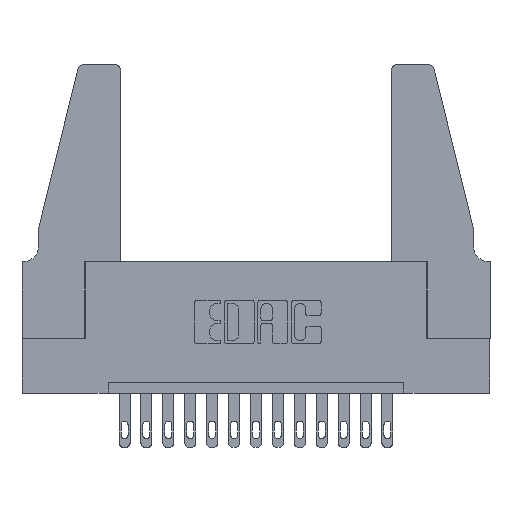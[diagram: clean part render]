
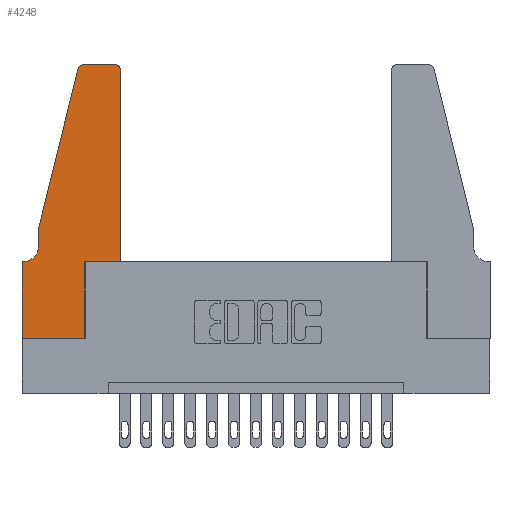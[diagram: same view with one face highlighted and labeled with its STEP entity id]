
A CAD part, top view. The second image highlights one B-rep face of the part: STEP entity #4248.
In plain terms, the highlighted planar face has unit normal (0, 0, 1).
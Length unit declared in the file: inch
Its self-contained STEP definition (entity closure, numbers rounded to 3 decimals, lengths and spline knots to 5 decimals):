
#276 = EDGE_CURVE ( 'NONE', #4902, #3095, #9481, .T. ) ;
#362 = CARTESIAN_POINT ( 'NONE',  ( 0.2605, 1.25, 0.37 ) ) ;
#485 = DIRECTION ( 'NONE',  ( 1., 0., 0. ) ) ;
#651 = CARTESIAN_POINT ( 'NONE',  ( 0.4505, 0.35, 0.37 ) ) ;
#668 = LINE ( 'NONE', #13694, #14025 ) ;
#690 = VECTOR ( 'NONE', #12337, 39.37008 ) ;
#999 = CARTESIAN_POINT ( 'NONE',  ( 0., 0., 0.37 ) ) ;
#1260 = CARTESIAN_POINT ( 'NONE',  ( 0.284, 1.25, 0.37 ) ) ;
#1362 = DIRECTION ( 'NONE',  ( 0., 0., 1. ) ) ;
#1658 = VERTEX_POINT ( 'NONE', #10302 ) ;
#1720 = ORIENTED_EDGE ( 'NONE', *, *, #7773, .T. ) ;
#1748 = VERTEX_POINT ( 'NONE', #2417 ) ;
#2011 = VECTOR ( 'NONE', #13747, 39.37008 ) ;
#2058 = VERTEX_POINT ( 'NONE', #1260 ) ;
#2111 = ORIENTED_EDGE ( 'NONE', *, *, #12207, .T. ) ;
#2129 = DIRECTION ( 'NONE',  ( 0., -1., 0. ) ) ;
#2417 = CARTESIAN_POINT ( 'NONE',  ( 0.0755, 0.5, 0.37 ) ) ;
#2458 = CARTESIAN_POINT ( 'NONE',  ( 0.2865, 0.35, 0.37 ) ) ;
#2506 = VERTEX_POINT ( 'NONE', #999 ) ;
#2629 = ORIENTED_EDGE ( 'NONE', *, *, #15460, .T. ) ;
#2761 = VERTEX_POINT ( 'NONE', #12954 ) ;
#2766 = AXIS2_PLACEMENT_3D ( 'NONE', #8630, #1362, #9855 ) ;
#3017 = AXIS2_PLACEMENT_3D ( 'NONE', #14844, #3873, #13804 ) ;
#3095 = VERTEX_POINT ( 'NONE', #2458 ) ;
#3340 = DIRECTION ( 'NONE',  ( 0., 1., 0. ) ) ;
#3521 = CARTESIAN_POINT ( 'NONE',  ( 0.0755, 0.5, 0.37 ) ) ;
#3535 = ORIENTED_EDGE ( 'NONE', *, *, #276, .T. ) ;
#3569 = ORIENTED_EDGE ( 'NONE', *, *, #9164, .T. ) ;
#3797 = VECTOR ( 'NONE', #12333, 39.37008 ) ;
#3873 = DIRECTION ( 'NONE',  ( 0., 0., -1. ) ) ;
#3899 = EDGE_CURVE ( 'NONE', #2506, #4902, #15775, .T. ) ;
#3939 = VECTOR ( 'NONE', #2129, 39.37008 ) ;
#4248 = ADVANCED_FACE ( 'NONE', ( #6786 ), #12271, .T. ) ;
#4289 = LINE ( 'NONE', #4987, #690 ) ;
#4370 = ORIENTED_EDGE ( 'NONE', *, *, #4925, .T. ) ;
#4902 = VERTEX_POINT ( 'NONE', #9717 ) ;
#4925 = EDGE_CURVE ( 'NONE', #12838, #2506, #4289, .T. ) ;
#4987 = CARTESIAN_POINT ( 'NONE',  ( 0., 0., 0.37 ) ) ;
#5018 = ORIENTED_EDGE ( 'NONE', *, *, #11725, .T. ) ;
#5132 = ORIENTED_EDGE ( 'NONE', *, *, #5438, .T. ) ;
#5137 = CIRCLE ( 'NONE', #13045, 0.03 ) ;
#5313 = CARTESIAN_POINT ( 'NONE',  ( 0.0755, 0.42, 0.37 ) ) ;
#5438 = EDGE_CURVE ( 'NONE', #15769, #1748, #11888, .T. ) ;
#5461 = LINE ( 'NONE', #9497, #3939 ) ;
#5871 = CARTESIAN_POINT ( 'NONE',  ( 0.2865, 0.35, 0.37 ) ) ;
#6216 = CARTESIAN_POINT ( 'NONE',  ( 0.0755, 0.35, 0.37 ) ) ;
#6357 = CARTESIAN_POINT ( 'NONE',  ( 0., 0.35, 0.37 ) ) ;
#6607 = VECTOR ( 'NONE', #10458, 39.37008 ) ;
#6786 = FACE_OUTER_BOUND ( 'NONE', #11342, .T. ) ;
#7773 = EDGE_CURVE ( 'NONE', #8274, #12838, #15400, .T. ) ;
#8274 = VERTEX_POINT ( 'NONE', #14135 ) ;
#8353 = EDGE_CURVE ( 'NONE', #12361, #8274, #15389, .T. ) ;
#8473 = CARTESIAN_POINT ( 'NONE',  ( 0.284, 1.22, 0.37 ) ) ;
#8630 = CARTESIAN_POINT ( 'NONE',  ( 0., 0.35, 0.37 ) ) ;
#8799 = DIRECTION ( 'NONE',  ( 1., 0., 0. ) ) ;
#8916 = DIRECTION ( 'NONE',  ( 0., 0., 1. ) ) ;
#8934 = AXIS2_PLACEMENT_3D ( 'NONE', #9027, #8916, #485 ) ;
#8951 = CARTESIAN_POINT ( 'NONE',  ( 0.4205, 1.25, 0.37 ) ) ;
#9027 = CARTESIAN_POINT ( 'NONE',  ( 0.4205, 1.22, 0.37 ) ) ;
#9164 = EDGE_CURVE ( 'NONE', #1658, #2761, #10565, .T. ) ;
#9481 = LINE ( 'NONE', #5871, #14838 ) ;
#9497 = CARTESIAN_POINT ( 'NONE',  ( 0.0755, 0.5, 0.37 ) ) ;
#9717 = CARTESIAN_POINT ( 'NONE',  ( 0.2865, 0., 0.37 ) ) ;
#9736 = EDGE_CURVE ( 'NONE', #3095, #1658, #668, .T. ) ;
#9794 = ORIENTED_EDGE ( 'NONE', *, *, #3899, .T. ) ;
#9803 = CARTESIAN_POINT ( 'NONE',  ( 0.25487, 1.22718, 0.37 ) ) ;
#9855 = DIRECTION ( 'NONE',  ( 1., 0., 0. ) ) ;
#10302 = CARTESIAN_POINT ( 'NONE',  ( 0.4505, 0.35, 0.37 ) ) ;
#10458 = DIRECTION ( 'NONE',  ( 1., 0., 0. ) ) ;
#10565 = LINE ( 'NONE', #651, #11163 ) ;
#11040 = DIRECTION ( 'NONE',  ( 1., 0., 0. ) ) ;
#11163 = VECTOR ( 'NONE', #12831, 39.37008 ) ;
#11342 = EDGE_LOOP ( 'NONE', ( #15385, #2111, #5132, #2629, #11492, #1720, #4370, #9794, #3535, #14359, #3569, #5018 ) ) ;
#11492 = ORIENTED_EDGE ( 'NONE', *, *, #8353, .T. ) ;
#11725 = EDGE_CURVE ( 'NONE', #2761, #13469, #12406, .T. ) ;
#11888 = LINE ( 'NONE', #3521, #2011 ) ;
#12162 = DIRECTION ( 'NONE',  ( 0., 0., 1. ) ) ;
#12207 = EDGE_CURVE ( 'NONE', #2058, #15769, #5137, .T. ) ;
#12271 = PLANE ( 'NONE',  #2766 ) ;
#12333 = DIRECTION ( 'NONE',  ( -1., 0., 0. ) ) ;
#12337 = DIRECTION ( 'NONE',  ( 0., -1., 0. ) ) ;
#12361 = VERTEX_POINT ( 'NONE', #5313 ) ;
#12406 = CIRCLE ( 'NONE', #8934, 0.03 ) ;
#12713 = CARTESIAN_POINT ( 'NONE',  ( 0., 0., 0.37 ) ) ;
#12779 = EDGE_CURVE ( 'NONE', #13469, #2058, #15448, .T. ) ;
#12831 = DIRECTION ( 'NONE',  ( 0., 1., 0. ) ) ;
#12838 = VERTEX_POINT ( 'NONE', #6357 ) ;
#12954 = CARTESIAN_POINT ( 'NONE',  ( 0.4505, 1.22, 0.37 ) ) ;
#13045 = AXIS2_PLACEMENT_3D ( 'NONE', #8473, #12162, #11040 ) ;
#13321 = VECTOR ( 'NONE', #14863, 39.37008 ) ;
#13469 = VERTEX_POINT ( 'NONE', #8951 ) ;
#13694 = CARTESIAN_POINT ( 'NONE',  ( 0.4505, 0.35, 0.37 ) ) ;
#13747 = DIRECTION ( 'NONE',  ( -0.239, -0.971, 0. ) ) ;
#13804 = DIRECTION ( 'NONE',  ( -1., 0., 0. ) ) ;
#14025 = VECTOR ( 'NONE', #8799, 39.37008 ) ;
#14135 = CARTESIAN_POINT ( 'NONE',  ( 0.0055, 0.35, 0.37 ) ) ;
#14359 = ORIENTED_EDGE ( 'NONE', *, *, #9736, .T. ) ;
#14838 = VECTOR ( 'NONE', #3340, 39.37008 ) ;
#14844 = CARTESIAN_POINT ( 'NONE',  ( 0.0055, 0.42, 0.37 ) ) ;
#14863 = DIRECTION ( 'NONE',  ( -1., 0., 0. ) ) ;
#15385 = ORIENTED_EDGE ( 'NONE', *, *, #12779, .T. ) ;
#15389 = CIRCLE ( 'NONE', #3017, 0.07 ) ;
#15400 = LINE ( 'NONE', #6216, #13321 ) ;
#15448 = LINE ( 'NONE', #362, #3797 ) ;
#15460 = EDGE_CURVE ( 'NONE', #1748, #12361, #5461, .T. ) ;
#15769 = VERTEX_POINT ( 'NONE', #9803 ) ;
#15775 = LINE ( 'NONE', #12713, #6607 ) ;
